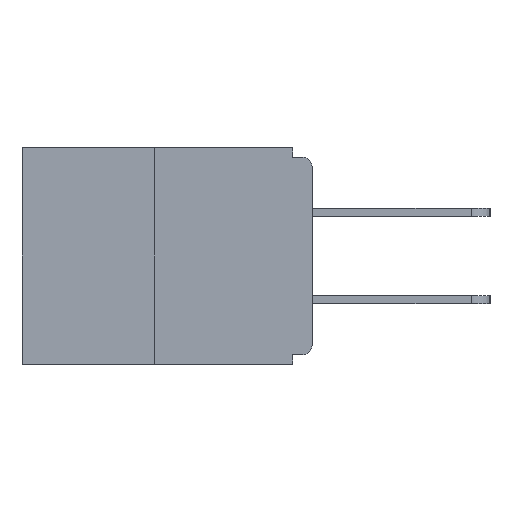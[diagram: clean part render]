
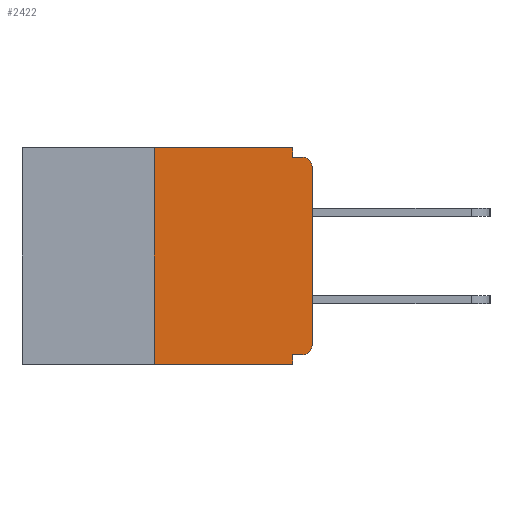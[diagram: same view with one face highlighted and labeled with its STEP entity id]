
A CAD part, left-side view. The second image highlights one B-rep face of the part: STEP entity #2422.
In plain terms, the highlighted planar face has unit normal (-1, 0, 0).
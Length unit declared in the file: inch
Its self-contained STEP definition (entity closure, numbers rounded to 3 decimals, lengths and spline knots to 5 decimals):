
#19 = CARTESIAN_POINT ( 'NONE',  ( 0., 0.25, 0. ) ) ;
#415 = ORIENTED_EDGE ( 'NONE', *, *, #3866, .F. ) ;
#521 = VERTEX_POINT ( 'NONE', #11827 ) ;
#781 = VECTOR ( 'NONE', #5756, 39.37008 ) ;
#963 = EDGE_CURVE ( 'NONE', #521, #14031, #3352, .T. ) ;
#1075 = CARTESIAN_POINT ( 'NONE',  ( 0., 0.015, -0.03 ) ) ;
#1369 = VECTOR ( 'NONE', #9517, 39.37008 ) ;
#1843 = LINE ( 'NONE', #16724, #781 ) ;
#1875 = VECTOR ( 'NONE', #9532, 39.37008 ) ;
#2081 = ORIENTED_EDGE ( 'NONE', *, *, #13010, .T. ) ;
#2115 = CARTESIAN_POINT ( 'NONE',  ( 0., 0., 0. ) ) ;
#2263 = DIRECTION ( 'NONE',  ( 0., 0., -1. ) ) ;
#2316 = DIRECTION ( 'NONE',  ( 0., 0., -1. ) ) ;
#2400 = CARTESIAN_POINT ( 'NONE',  ( 0., 0.031, 0. ) ) ;
#2422 = ADVANCED_FACE ( 'NONE', ( #16388 ), #13382, .F. ) ;
#3006 = DIRECTION ( 'NONE',  ( 0., -1., 0. ) ) ;
#3194 = VECTOR ( 'NONE', #11584, 39.37008 ) ;
#3332 = CIRCLE ( 'NONE', #11856, 0.015 ) ;
#3352 = CIRCLE ( 'NONE', #17076, 0.015 ) ;
#3553 = LINE ( 'NONE', #4549, #15029 ) ;
#3866 = EDGE_CURVE ( 'NONE', #10287, #6514, #6130, .T. ) ;
#3920 = LINE ( 'NONE', #17451, #7707 ) ;
#4056 = VERTEX_POINT ( 'NONE', #8572 ) ;
#4163 = CARTESIAN_POINT ( 'NONE',  ( 0., 0.46, 0. ) ) ;
#4334 = DIRECTION ( 'NONE',  ( 0., 0., -1. ) ) ;
#4390 = DIRECTION ( 'NONE',  ( 0., 0., -1. ) ) ;
#4549 = CARTESIAN_POINT ( 'NONE',  ( 0., 0.031, -0.343 ) ) ;
#4689 = LINE ( 'NONE', #2115, #3194 ) ;
#4691 = CARTESIAN_POINT ( 'NONE',  ( 0., 0.031, 0. ) ) ;
#5280 = DIRECTION ( 'NONE',  ( 0., 0., -1. ) ) ;
#5756 = DIRECTION ( 'NONE',  ( 0., -1., 0. ) ) ;
#6130 = LINE ( 'NONE', #19, #1875 ) ;
#6253 = VERTEX_POINT ( 'NONE', #9092 ) ;
#6514 = VERTEX_POINT ( 'NONE', #11065 ) ;
#6629 = CARTESIAN_POINT ( 'NONE',  ( 0., 0.031, -0.015 ) ) ;
#6725 = CARTESIAN_POINT ( 'NONE',  ( 0., 0.015, -0.313 ) ) ;
#7419 = VECTOR ( 'NONE', #8681, 39.37008 ) ;
#7423 = CARTESIAN_POINT ( 'NONE',  ( 0., 0., -0.328 ) ) ;
#7473 = VERTEX_POINT ( 'NONE', #4691 ) ;
#7707 = VECTOR ( 'NONE', #3006, 39.37008 ) ;
#8135 = AXIS2_PLACEMENT_3D ( 'NONE', #4163, #9550, #4334 ) ;
#8469 = ORIENTED_EDGE ( 'NONE', *, *, #9394, .F. ) ;
#8572 = CARTESIAN_POINT ( 'NONE',  ( 0., 0.015, -0.015 ) ) ;
#8681 = DIRECTION ( 'NONE',  ( 0., 1., 0. ) ) ;
#8987 = DIRECTION ( 'NONE',  ( -1., 0., 0. ) ) ;
#9092 = CARTESIAN_POINT ( 'NONE',  ( 0., 0., -0.03 ) ) ;
#9394 = EDGE_CURVE ( 'NONE', #15523, #4056, #1843, .T. ) ;
#9490 = EDGE_CURVE ( 'NONE', #16046, #17302, #3553, .T. ) ;
#9517 = DIRECTION ( 'NONE',  ( 0., -1., 0. ) ) ;
#9532 = DIRECTION ( 'NONE',  ( 0., 0., 1. ) ) ;
#9550 = DIRECTION ( 'NONE',  ( 1., 0., 0. ) ) ;
#10287 = VERTEX_POINT ( 'NONE', #17485 ) ;
#10888 = EDGE_CURVE ( 'NONE', #6514, #7473, #14757, .T. ) ;
#11001 = LINE ( 'NONE', #7423, #7419 ) ;
#11065 = CARTESIAN_POINT ( 'NONE',  ( 0., 0.25, 0. ) ) ;
#11584 = DIRECTION ( 'NONE',  ( 0., 0., 1. ) ) ;
#11827 = CARTESIAN_POINT ( 'NONE',  ( 0., 0.015, -0.328 ) ) ;
#11856 = AXIS2_PLACEMENT_3D ( 'NONE', #1075, #13118, #2316 ) ;
#11988 = ORIENTED_EDGE ( 'NONE', *, *, #16886, .T. ) ;
#12171 = ORIENTED_EDGE ( 'NONE', *, *, #963, .T. ) ;
#12408 = VECTOR ( 'NONE', #5280, 39.37008 ) ;
#12532 = EDGE_LOOP ( 'NONE', ( #14135, #415, #11988, #17425, #17511, #12171, #2081, #17474, #8469, #14372 ) ) ;
#13010 = EDGE_CURVE ( 'NONE', #14031, #6253, #4689, .T. ) ;
#13118 = DIRECTION ( 'NONE',  ( -1., 0., 0. ) ) ;
#13246 = LINE ( 'NONE', #2400, #12408 ) ;
#13382 = PLANE ( 'NONE',  #8135 ) ;
#13405 = CARTESIAN_POINT ( 'NONE',  ( 0., 0.46, 0. ) ) ;
#13970 = CARTESIAN_POINT ( 'NONE',  ( 0., 0.031, -0.343 ) ) ;
#14031 = VERTEX_POINT ( 'NONE', #14804 ) ;
#14135 = ORIENTED_EDGE ( 'NONE', *, *, #10888, .F. ) ;
#14328 = EDGE_CURVE ( 'NONE', #521, #16046, #11001, .T. ) ;
#14372 = ORIENTED_EDGE ( 'NONE', *, *, #16337, .F. ) ;
#14757 = LINE ( 'NONE', #13405, #1369 ) ;
#14804 = CARTESIAN_POINT ( 'NONE',  ( 0., 0., -0.313 ) ) ;
#14886 = EDGE_CURVE ( 'NONE', #6253, #4056, #3332, .T. ) ;
#15029 = VECTOR ( 'NONE', #4390, 39.37008 ) ;
#15523 = VERTEX_POINT ( 'NONE', #6629 ) ;
#16046 = VERTEX_POINT ( 'NONE', #16584 ) ;
#16337 = EDGE_CURVE ( 'NONE', #7473, #15523, #13246, .T. ) ;
#16388 = FACE_OUTER_BOUND ( 'NONE', #12532, .T. ) ;
#16584 = CARTESIAN_POINT ( 'NONE',  ( 0., 0.031, -0.328 ) ) ;
#16724 = CARTESIAN_POINT ( 'NONE',  ( 0., 0., -0.015 ) ) ;
#16886 = EDGE_CURVE ( 'NONE', #10287, #17302, #3920, .T. ) ;
#17076 = AXIS2_PLACEMENT_3D ( 'NONE', #6725, #8987, #2263 ) ;
#17302 = VERTEX_POINT ( 'NONE', #13970 ) ;
#17425 = ORIENTED_EDGE ( 'NONE', *, *, #9490, .F. ) ;
#17451 = CARTESIAN_POINT ( 'NONE',  ( 0., 0.46, -0.343 ) ) ;
#17474 = ORIENTED_EDGE ( 'NONE', *, *, #14886, .T. ) ;
#17485 = CARTESIAN_POINT ( 'NONE',  ( 0., 0.25, -0.343 ) ) ;
#17511 = ORIENTED_EDGE ( 'NONE', *, *, #14328, .F. ) ;
